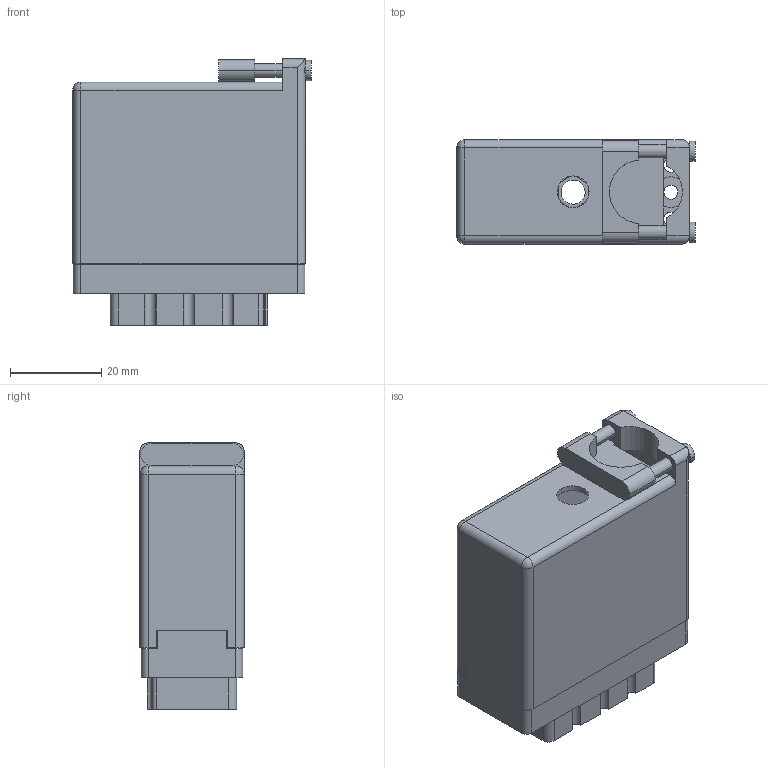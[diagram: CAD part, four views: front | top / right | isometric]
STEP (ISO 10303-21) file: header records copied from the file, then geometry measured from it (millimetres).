
FILE_DESCRIPTION (( 'STEP AP203' ), '1' );
FILE_NAME ('516-038-000-460.STEP', '2020-03-04T22:05:47', ( '' ), ( '' ), 'SwSTEP 2.0', 'SolidWorks 2016', '' );
FILE_SCHEMA (( 'CONFIG_CONTROL_DESIGN' ));
Length unit declared in the file: inch
Products named in the file (3): 516-038-000-460; 516-230-001_Metal - 038 Top Entry; 516 Part Receptacle_038
Assembly tree (2 placements, depth 2):
  516-038-000-460
    516 Part Receptacle_038
    516-230-001_Metal - 038 Top Entry
Bounding box: 52.27 x 22.83 x 58.34 mm (x, y, z)
Volume: 19623.8 mm3; surface area: 28585.3 mm2
Topology: 2 solids, 2 shells, 980 faces, 2872 edges, 1908 vertices
Faces by surface type: plane 670, cylinder 306, cone 2, sphere 2
Entity records: 33090 total; most frequent: CARTESIAN_POINT 5805, ORIENTED_EDGE 5740, DIRECTION 5599, EDGE_CURVE 2870, VECTOR 2099, LINE 2099, VERTEX_POINT 1908, AXIS2_PLACEMENT_3D 1750
